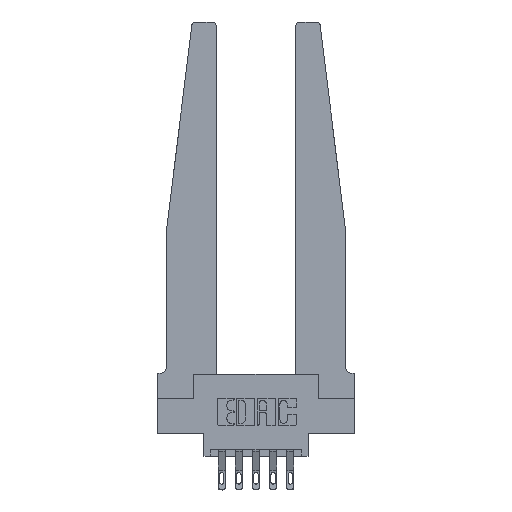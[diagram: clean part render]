
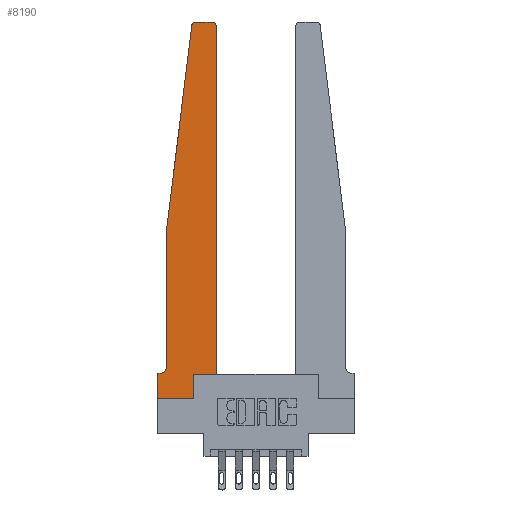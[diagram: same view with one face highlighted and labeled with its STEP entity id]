
A CAD part, top view. The second image highlights one B-rep face of the part: STEP entity #8190.
In plain terms, the highlighted planar face has unit normal (0, 0, 1).
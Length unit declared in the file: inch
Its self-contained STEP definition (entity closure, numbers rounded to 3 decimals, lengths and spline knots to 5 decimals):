
#44 = DIRECTION ( 'NONE',  ( 1., 0., 0. ) ) ;
#134 = CARTESIAN_POINT ( 'NONE',  ( 0.065, 0.2375, 0.37 ) ) ;
#717 = EDGE_CURVE ( 'NONE', #10484, #4092, #11706, .T. ) ;
#830 = ORIENTED_EDGE ( 'NONE', *, *, #13728, .T. ) ;
#871 = DIRECTION ( 'NONE',  ( 1., 0., 0. ) ) ;
#952 = ORIENTED_EDGE ( 'NONE', *, *, #1096, .T. ) ;
#1077 = ORIENTED_EDGE ( 'NONE', *, *, #6544, .T. ) ;
#1096 = EDGE_CURVE ( 'NONE', #4288, #8885, #6487, .T. ) ;
#1216 = VECTOR ( 'NONE', #6288, 39.37008 ) ;
#1431 = ORIENTED_EDGE ( 'NONE', *, *, #6563, .T. ) ;
#1641 = CARTESIAN_POINT ( 'NONE',  ( 0.2605, 0., 0.37 ) ) ;
#1684 = VECTOR ( 'NONE', #9517, 39.37008 ) ;
#1922 = EDGE_CURVE ( 'NONE', #10965, #10484, #8916, .T. ) ;
#2132 = EDGE_CURVE ( 'NONE', #9633, #4288, #12668, .T. ) ;
#2163 = VERTEX_POINT ( 'NONE', #13372 ) ;
#2445 = LINE ( 'NONE', #3499, #12018 ) ;
#2564 = CARTESIAN_POINT ( 'NONE',  ( 0.425, 2.72, 0.37 ) ) ;
#2680 = EDGE_LOOP ( 'NONE', ( #12319, #4211, #952, #10709, #1431, #9551, #8601, #3735, #6325, #1077, #7973, #830 ) ) ;
#2738 = VECTOR ( 'NONE', #8544, 39.37008 ) ;
#2846 = LINE ( 'NONE', #9395, #1684 ) ;
#2917 = CARTESIAN_POINT ( 'NONE',  ( 0.27653, 2.72, 0.37 ) ) ;
#3046 = CIRCLE ( 'NONE', #10224, 0.05 ) ;
#3157 = LINE ( 'NONE', #6386, #7326 ) ;
#3168 = EDGE_CURVE ( 'NONE', #10258, #2163, #3157, .T. ) ;
#3289 = DIRECTION ( 'NONE',  ( 0., 0., -1. ) ) ;
#3402 = VERTEX_POINT ( 'NONE', #11501 ) ;
#3499 = CARTESIAN_POINT ( 'NONE',  ( 0.425, 0.18, 0.37 ) ) ;
#3504 = CARTESIAN_POINT ( 'NONE',  ( 0.065, 0.1875, 0.37 ) ) ;
#3539 = VECTOR ( 'NONE', #8940, 39.37008 ) ;
#3735 = ORIENTED_EDGE ( 'NONE', *, *, #8424, .T. ) ;
#4092 = VERTEX_POINT ( 'NONE', #11901 ) ;
#4177 = DIRECTION ( 'NONE',  ( -0.122, -0.992, 0. ) ) ;
#4211 = ORIENTED_EDGE ( 'NONE', *, *, #2132, .T. ) ;
#4269 = CARTESIAN_POINT ( 'NONE',  ( 0.015, 0.2375, 0.37 ) ) ;
#4288 = VERTEX_POINT ( 'NONE', #7537 ) ;
#4330 = DIRECTION ( 'NONE',  ( -1., 0., 0. ) ) ;
#4360 = AXIS2_PLACEMENT_3D ( 'NONE', #2917, #7213, #871 ) ;
#4695 = CARTESIAN_POINT ( 'NONE',  ( 0.015, 0.1875, 0.37 ) ) ;
#5495 = CARTESIAN_POINT ( 'NONE',  ( 0., 0.1875, 0.37 ) ) ;
#6007 = VERTEX_POINT ( 'NONE', #134 ) ;
#6090 = LINE ( 'NONE', #12621, #12286 ) ;
#6194 = CIRCLE ( 'NONE', #13605, 0.03 ) ;
#6288 = DIRECTION ( 'NONE',  ( -1., 0., 0. ) ) ;
#6325 = ORIENTED_EDGE ( 'NONE', *, *, #3168, .T. ) ;
#6361 = VECTOR ( 'NONE', #13199, 39.37008 ) ;
#6386 = CARTESIAN_POINT ( 'NONE',  ( 0.2605, 0.18, 0.37 ) ) ;
#6487 = LINE ( 'NONE', #13820, #9034 ) ;
#6544 = EDGE_CURVE ( 'NONE', #2163, #3402, #2445, .T. ) ;
#6563 = EDGE_CURVE ( 'NONE', #6007, #10965, #3046, .T. ) ;
#6680 = DIRECTION ( 'NONE',  ( 1., 0., 0. ) ) ;
#7067 = AXIS2_PLACEMENT_3D ( 'NONE', #11980, #8611, #7695 ) ;
#7213 = DIRECTION ( 'NONE',  ( 0., 0., 1. ) ) ;
#7326 = VECTOR ( 'NONE', #13783, 39.37008 ) ;
#7537 = CARTESIAN_POINT ( 'NONE',  ( 0.24675, 2.72367, 0.37 ) ) ;
#7576 = FACE_OUTER_BOUND ( 'NONE', #2680, .T. ) ;
#7603 = CARTESIAN_POINT ( 'NONE',  ( 0.395, 2.72, 0.37 ) ) ;
#7673 = CARTESIAN_POINT ( 'NONE',  ( 0.425, 0.18, 0.37 ) ) ;
#7695 = DIRECTION ( 'NONE',  ( 1., 0., 0. ) ) ;
#7973 = ORIENTED_EDGE ( 'NONE', *, *, #13282, .T. ) ;
#8190 = ADVANCED_FACE ( 'NONE', ( #7576 ), #13108, .T. ) ;
#8424 = EDGE_CURVE ( 'NONE', #4092, #10258, #2846, .T. ) ;
#8544 = DIRECTION ( 'NONE',  ( 0., -1., 0. ) ) ;
#8601 = ORIENTED_EDGE ( 'NONE', *, *, #717, .T. ) ;
#8610 = CARTESIAN_POINT ( 'NONE',  ( 0., 0., 0.37 ) ) ;
#8611 = DIRECTION ( 'NONE',  ( 0., 0., 1. ) ) ;
#8873 = LINE ( 'NONE', #7673, #3539 ) ;
#8885 = VERTEX_POINT ( 'NONE', #13053 ) ;
#8916 = LINE ( 'NONE', #3504, #6361 ) ;
#8940 = DIRECTION ( 'NONE',  ( 0., 1., 0. ) ) ;
#9034 = VECTOR ( 'NONE', #4177, 39.37008 ) ;
#9347 = VERTEX_POINT ( 'NONE', #2564 ) ;
#9395 = CARTESIAN_POINT ( 'NONE',  ( 0., 0., 0.37 ) ) ;
#9517 = DIRECTION ( 'NONE',  ( 1., 0., 0. ) ) ;
#9521 = EDGE_CURVE ( 'NONE', #12639, #9633, #12614, .T. ) ;
#9551 = ORIENTED_EDGE ( 'NONE', *, *, #1922, .T. ) ;
#9633 = VERTEX_POINT ( 'NONE', #12962 ) ;
#9969 = DIRECTION ( 'NONE',  ( 0., 0., 1. ) ) ;
#10224 = AXIS2_PLACEMENT_3D ( 'NONE', #4269, #3289, #4330 ) ;
#10258 = VERTEX_POINT ( 'NONE', #1641 ) ;
#10370 = DIRECTION ( 'NONE',  ( 0., -1., 0. ) ) ;
#10436 = CARTESIAN_POINT ( 'NONE',  ( 0.25, 2.75, 0.37 ) ) ;
#10484 = VERTEX_POINT ( 'NONE', #5495 ) ;
#10709 = ORIENTED_EDGE ( 'NONE', *, *, #12669, .T. ) ;
#10965 = VERTEX_POINT ( 'NONE', #4695 ) ;
#11501 = CARTESIAN_POINT ( 'NONE',  ( 0.425, 0.18, 0.37 ) ) ;
#11706 = LINE ( 'NONE', #8610, #2738 ) ;
#11901 = CARTESIAN_POINT ( 'NONE',  ( 0., 0., 0.37 ) ) ;
#11980 = CARTESIAN_POINT ( 'NONE',  ( 0., 0.1875, 0.37 ) ) ;
#12018 = VECTOR ( 'NONE', #44, 39.37008 ) ;
#12286 = VECTOR ( 'NONE', #10370, 39.37008 ) ;
#12319 = ORIENTED_EDGE ( 'NONE', *, *, #9521, .T. ) ;
#12489 = CARTESIAN_POINT ( 'NONE',  ( 0.395, 2.75, 0.37 ) ) ;
#12614 = LINE ( 'NONE', #10436, #1216 ) ;
#12621 = CARTESIAN_POINT ( 'NONE',  ( 0.065, 1.25, 0.37 ) ) ;
#12639 = VERTEX_POINT ( 'NONE', #12489 ) ;
#12668 = CIRCLE ( 'NONE', #4360, 0.03 ) ;
#12669 = EDGE_CURVE ( 'NONE', #8885, #6007, #6090, .T. ) ;
#12962 = CARTESIAN_POINT ( 'NONE',  ( 0.27653, 2.75, 0.37 ) ) ;
#13053 = CARTESIAN_POINT ( 'NONE',  ( 0.065, 1.25, 0.37 ) ) ;
#13108 = PLANE ( 'NONE',  #7067 ) ;
#13199 = DIRECTION ( 'NONE',  ( -1., 0., 0. ) ) ;
#13282 = EDGE_CURVE ( 'NONE', #3402, #9347, #8873, .T. ) ;
#13372 = CARTESIAN_POINT ( 'NONE',  ( 0.2605, 0.18, 0.37 ) ) ;
#13605 = AXIS2_PLACEMENT_3D ( 'NONE', #7603, #9969, #6680 ) ;
#13728 = EDGE_CURVE ( 'NONE', #9347, #12639, #6194, .T. ) ;
#13783 = DIRECTION ( 'NONE',  ( 0., 1., 0. ) ) ;
#13820 = CARTESIAN_POINT ( 'NONE',  ( 0.065, 1.25, 0.37 ) ) ;
